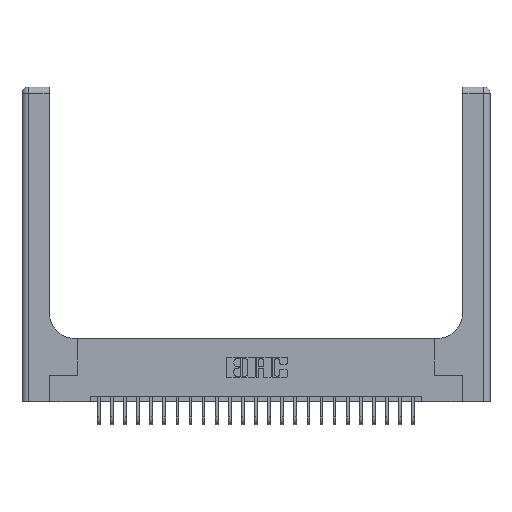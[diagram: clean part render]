
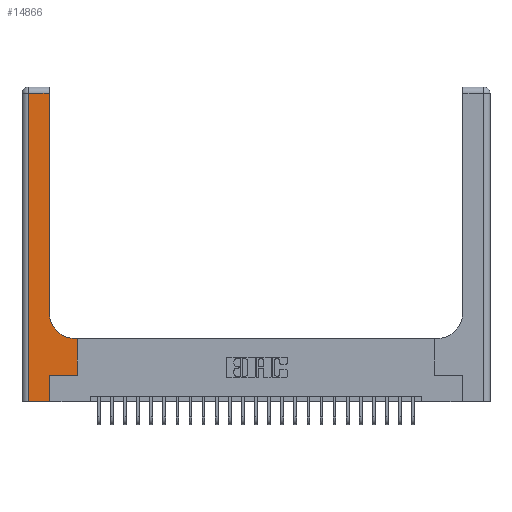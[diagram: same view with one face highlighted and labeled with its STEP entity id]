
A CAD part, top view. The second image highlights one B-rep face of the part: STEP entity #14866.
In plain terms, the highlighted planar face has unit normal (0, 0, 1).
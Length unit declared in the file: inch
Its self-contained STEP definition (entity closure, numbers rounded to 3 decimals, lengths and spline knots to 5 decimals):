
#1332 = DIRECTION ( 'NONE',  ( 0., -1., 0. ) ) ;
#1359 = DIRECTION ( 'NONE',  ( -1., 0., 0. ) ) ;
#1589 = VERTEX_POINT ( 'NONE', #7076 ) ;
#1841 = LINE ( 'NONE', #15958, #15717 ) ;
#2356 = EDGE_CURVE ( 'NONE', #12714, #17747, #19197, .T. ) ;
#2628 = VERTEX_POINT ( 'NONE', #14776 ) ;
#2907 = DIRECTION ( 'NONE',  ( 0., 1., 0. ) ) ;
#2920 = ORIENTED_EDGE ( 'NONE', *, *, #24829, .T. ) ;
#3149 = LINE ( 'NONE', #4775, #22299 ) ;
#3230 = CARTESIAN_POINT ( 'NONE',  ( 0.06, 3., 0.37 ) ) ;
#3488 = ORIENTED_EDGE ( 'NONE', *, *, #2356, .T. ) ;
#3780 = CARTESIAN_POINT ( 'NONE',  ( 0.26, 0.6, 0.37 ) ) ;
#4226 = DIRECTION ( 'NONE',  ( 0., 0., -1. ) ) ;
#4605 = CARTESIAN_POINT ( 'NONE',  ( 0.265, 0.25, 0.37 ) ) ;
#4717 = CARTESIAN_POINT ( 'NONE',  ( 0.06, 0., 0.37 ) ) ;
#4775 = CARTESIAN_POINT ( 'NONE',  ( 0.528, 0.25, 0.37 ) ) ;
#4803 = EDGE_CURVE ( 'NONE', #2628, #5493, #3149, .T. ) ;
#4963 = LINE ( 'NONE', #10567, #23856 ) ;
#5451 = VERTEX_POINT ( 'NONE', #16263 ) ;
#5493 = VERTEX_POINT ( 'NONE', #8626 ) ;
#5625 = CIRCLE ( 'NONE', #10165, 0.25 ) ;
#7076 = CARTESIAN_POINT ( 'NONE',  ( 0.265, 0., 0.37 ) ) ;
#7976 = DIRECTION ( 'NONE',  ( 0., 1., 0. ) ) ;
#8454 = CARTESIAN_POINT ( 'NONE',  ( 0., 3., 0.37 ) ) ;
#8607 = DIRECTION ( 'NONE',  ( -1., 0., 0. ) ) ;
#8626 = CARTESIAN_POINT ( 'NONE',  ( 0.528, 0.6, 0.37 ) ) ;
#8692 = CARTESIAN_POINT ( 'NONE',  ( 0., 2.94, 0.37 ) ) ;
#9244 = VECTOR ( 'NONE', #1332, 39.37008 ) ;
#9255 = EDGE_CURVE ( 'NONE', #12815, #14480, #5625, .T. ) ;
#10140 = VECTOR ( 'NONE', #1359, 39.37008 ) ;
#10165 = AXIS2_PLACEMENT_3D ( 'NONE', #16064, #4226, #18054 ) ;
#10215 = VECTOR ( 'NONE', #15417, 39.37008 ) ;
#10303 = ORIENTED_EDGE ( 'NONE', *, *, #12865, .T. ) ;
#10335 = ORIENTED_EDGE ( 'NONE', *, *, #4803, .T. ) ;
#10512 = VECTOR ( 'NONE', #8607, 39.37008 ) ;
#10567 = CARTESIAN_POINT ( 'NONE',  ( 0., 0., 0.37 ) ) ;
#10777 = LINE ( 'NONE', #3780, #10140 ) ;
#10912 = DIRECTION ( 'NONE',  ( 1., 0., 0. ) ) ;
#11960 = LINE ( 'NONE', #22895, #22798 ) ;
#12686 = VERTEX_POINT ( 'NONE', #4605 ) ;
#12714 = VERTEX_POINT ( 'NONE', #21035 ) ;
#12815 = VERTEX_POINT ( 'NONE', #13152 ) ;
#12865 = EDGE_CURVE ( 'NONE', #1589, #12686, #19517, .T. ) ;
#13152 = CARTESIAN_POINT ( 'NONE',  ( 0.51, 0.6, 0.37 ) ) ;
#13741 = EDGE_LOOP ( 'NONE', ( #16341, #2920, #3488, #18078, #10303, #24349, #10335, #17561, #23762 ) ) ;
#14160 = EDGE_CURVE ( 'NONE', #5493, #12815, #10777, .T. ) ;
#14480 = VERTEX_POINT ( 'NONE', #25519 ) ;
#14776 = CARTESIAN_POINT ( 'NONE',  ( 0.528, 0.25, 0.37 ) ) ;
#14866 = ADVANCED_FACE ( 'NONE', ( #24072 ), #24172, .F. ) ;
#15089 = DIRECTION ( 'NONE',  ( -1., 0., 0. ) ) ;
#15417 = DIRECTION ( 'NONE',  ( 0., 1., 0. ) ) ;
#15717 = VECTOR ( 'NONE', #7976, 39.37008 ) ;
#15958 = CARTESIAN_POINT ( 'NONE',  ( 0.26, 3., 0.37 ) ) ;
#16064 = CARTESIAN_POINT ( 'NONE',  ( 0.51, 0.85, 0.37 ) ) ;
#16263 = CARTESIAN_POINT ( 'NONE',  ( 0.26, 2.94, 0.37 ) ) ;
#16341 = ORIENTED_EDGE ( 'NONE', *, *, #20521, .T. ) ;
#17561 = ORIENTED_EDGE ( 'NONE', *, *, #14160, .T. ) ;
#17747 = VERTEX_POINT ( 'NONE', #4717 ) ;
#18054 = DIRECTION ( 'NONE',  ( 1., 0., 0. ) ) ;
#18078 = ORIENTED_EDGE ( 'NONE', *, *, #24131, .T. ) ;
#19197 = LINE ( 'NONE', #3230, #9244 ) ;
#19415 = AXIS2_PLACEMENT_3D ( 'NONE', #8454, #24601, #15089 ) ;
#19517 = LINE ( 'NONE', #21310, #10215 ) ;
#20521 = EDGE_CURVE ( 'NONE', #14480, #5451, #1841, .T. ) ;
#21021 = EDGE_CURVE ( 'NONE', #12686, #2628, #11960, .T. ) ;
#21035 = CARTESIAN_POINT ( 'NONE',  ( 0.06, 2.94, 0.37 ) ) ;
#21310 = CARTESIAN_POINT ( 'NONE',  ( 0.265, 0., 0.37 ) ) ;
#22299 = VECTOR ( 'NONE', #2907, 39.37008 ) ;
#22798 = VECTOR ( 'NONE', #23140, 39.37008 ) ;
#22895 = CARTESIAN_POINT ( 'NONE',  ( 0.265, 0.25, 0.37 ) ) ;
#23140 = DIRECTION ( 'NONE',  ( 1., 0., 0. ) ) ;
#23762 = ORIENTED_EDGE ( 'NONE', *, *, #9255, .T. ) ;
#23856 = VECTOR ( 'NONE', #10912, 39.37008 ) ;
#24072 = FACE_OUTER_BOUND ( 'NONE', #13741, .T. ) ;
#24131 = EDGE_CURVE ( 'NONE', #17747, #1589, #4963, .T. ) ;
#24151 = LINE ( 'NONE', #8692, #10512 ) ;
#24172 = PLANE ( 'NONE',  #19415 ) ;
#24349 = ORIENTED_EDGE ( 'NONE', *, *, #21021, .T. ) ;
#24601 = DIRECTION ( 'NONE',  ( 0., 0., -1. ) ) ;
#24829 = EDGE_CURVE ( 'NONE', #5451, #12714, #24151, .T. ) ;
#25519 = CARTESIAN_POINT ( 'NONE',  ( 0.26, 0.85, 0.37 ) ) ;
